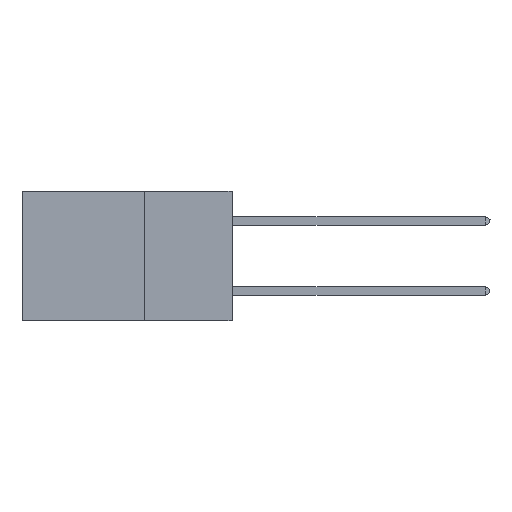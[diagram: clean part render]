
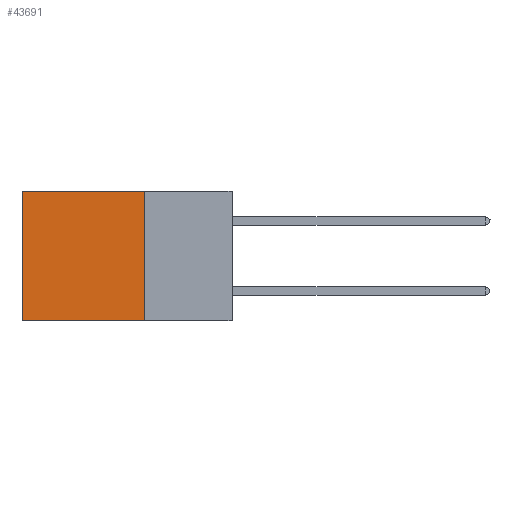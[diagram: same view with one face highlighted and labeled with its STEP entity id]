
A CAD part, left-side view. The second image highlights one B-rep face of the part: STEP entity #43691.
In plain terms, the highlighted planar face has unit normal (-1, 0, 0).
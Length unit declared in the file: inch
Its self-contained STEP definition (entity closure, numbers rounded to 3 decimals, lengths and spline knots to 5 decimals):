
#26 = DIRECTION ( 'NONE',  ( 0., 0., -1. ) ) ;
#969 = VECTOR ( 'NONE', #29332, 39.37008 ) ;
#986 = CARTESIAN_POINT ( 'NONE',  ( 0.2875, 0.6, 0. ) ) ;
#2668 = VERTEX_POINT ( 'NONE', #13638 ) ;
#3251 = DIRECTION ( 'NONE',  ( 1., 0., 0. ) ) ;
#3435 = LINE ( 'NONE', #27220, #30967 ) ;
#8347 = CARTESIAN_POINT ( 'NONE',  ( 0.2875, 0.25, 0. ) ) ;
#10539 = CARTESIAN_POINT ( 'NONE',  ( 0.2875, 0.25, 0. ) ) ;
#12239 = VERTEX_POINT ( 'NONE', #27405 ) ;
#12783 = EDGE_LOOP ( 'NONE', ( #28612, #41255, #20423, #13503 ) ) ;
#13503 = ORIENTED_EDGE ( 'NONE', *, *, #32673, .T. ) ;
#13638 = CARTESIAN_POINT ( 'NONE',  ( 0.2875, 0.6, 0. ) ) ;
#14465 = VECTOR ( 'NONE', #21842, 39.37008 ) ;
#16027 = VERTEX_POINT ( 'NONE', #10539 ) ;
#19107 = EDGE_CURVE ( 'NONE', #2668, #12239, #32296, .T. ) ;
#19459 = DIRECTION ( 'NONE',  ( 0., 1., 0. ) ) ;
#20423 = ORIENTED_EDGE ( 'NONE', *, *, #41640, .F. ) ;
#20607 = PLANE ( 'NONE',  #37202 ) ;
#21842 = DIRECTION ( 'NONE',  ( 0., 0., -1. ) ) ;
#23483 = CARTESIAN_POINT ( 'NONE',  ( 0.2875, 0.25, -0.37 ) ) ;
#23889 = VECTOR ( 'NONE', #19459, 39.37008 ) ;
#25276 = CARTESIAN_POINT ( 'NONE',  ( 0.2875, 0.25, 0. ) ) ;
#27132 = EDGE_CURVE ( 'NONE', #35100, #12239, #3435, .T. ) ;
#27220 = CARTESIAN_POINT ( 'NONE',  ( 0.2875, 0.25, -0.37 ) ) ;
#27405 = CARTESIAN_POINT ( 'NONE',  ( 0.2875, 0.6, -0.37 ) ) ;
#27919 = CARTESIAN_POINT ( 'NONE',  ( 0.2875, 0.25, 0. ) ) ;
#28612 = ORIENTED_EDGE ( 'NONE', *, *, #19107, .T. ) ;
#29332 = DIRECTION ( 'NONE',  ( 0., 0., -1. ) ) ;
#30967 = VECTOR ( 'NONE', #34514, 39.37008 ) ;
#31337 = FACE_OUTER_BOUND ( 'NONE', #12783, .T. ) ;
#32296 = LINE ( 'NONE', #986, #969 ) ;
#32673 = EDGE_CURVE ( 'NONE', #16027, #2668, #39622, .T. ) ;
#34514 = DIRECTION ( 'NONE',  ( 0., 1., 0. ) ) ;
#35100 = VERTEX_POINT ( 'NONE', #23483 ) ;
#37202 = AXIS2_PLACEMENT_3D ( 'NONE', #27919, #3251, #26 ) ;
#39622 = LINE ( 'NONE', #8347, #23889 ) ;
#41255 = ORIENTED_EDGE ( 'NONE', *, *, #27132, .F. ) ;
#41640 = EDGE_CURVE ( 'NONE', #16027, #35100, #42620, .T. ) ;
#42620 = LINE ( 'NONE', #25276, #14465 ) ;
#43691 = ADVANCED_FACE ( 'NONE', ( #31337 ), #20607, .F. ) ;
